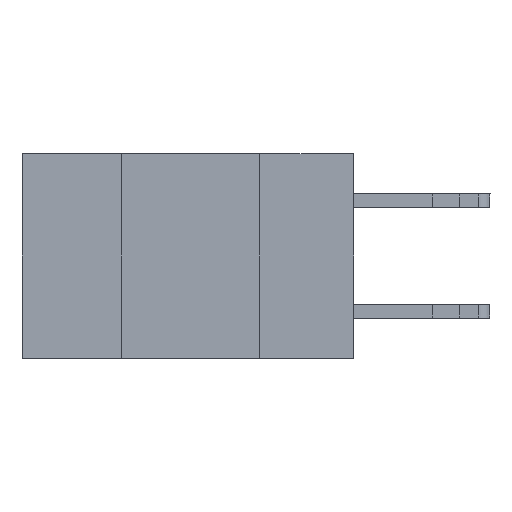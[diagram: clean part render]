
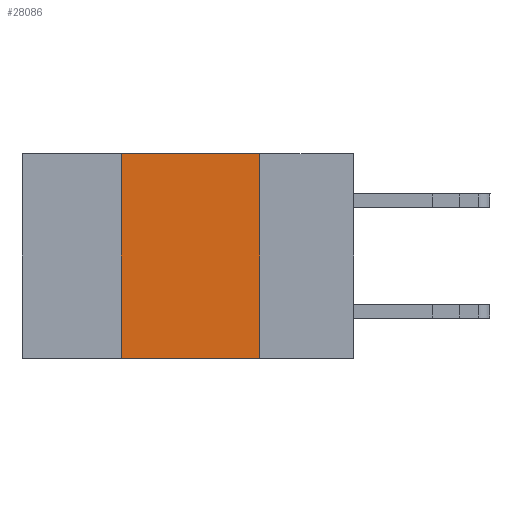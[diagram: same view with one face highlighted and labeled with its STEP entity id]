
A CAD part, left-side view. The second image highlights one B-rep face of the part: STEP entity #28086.
In plain terms, the highlighted planar face has unit normal (-1, 0, 0).
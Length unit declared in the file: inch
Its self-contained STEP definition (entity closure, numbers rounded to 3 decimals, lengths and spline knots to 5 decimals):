
#154 = DIRECTION ( 'NONE',  ( 0., -1., 0. ) ) ;
#2902 = CARTESIAN_POINT ( 'NONE',  ( 0., 0.17, 0. ) ) ;
#4293 = VERTEX_POINT ( 'NONE', #5622 ) ;
#4995 = DIRECTION ( 'NONE',  ( 0., 0., -1. ) ) ;
#5622 = CARTESIAN_POINT ( 'NONE',  ( 0., 0.42, 0. ) ) ;
#5686 = CARTESIAN_POINT ( 'NONE',  ( 0., 0.6, 0. ) ) ;
#6970 = VECTOR ( 'NONE', #25527, 39.37008 ) ;
#7393 = ORIENTED_EDGE ( 'NONE', *, *, #28038, .T. ) ;
#7588 = FACE_OUTER_BOUND ( 'NONE', #10348, .T. ) ;
#8051 = EDGE_CURVE ( 'NONE', #32552, #4293, #31285, .T. ) ;
#8640 = VERTEX_POINT ( 'NONE', #2902 ) ;
#9148 = AXIS2_PLACEMENT_3D ( 'NONE', #15513, #18278, #4995 ) ;
#9192 = ORIENTED_EDGE ( 'NONE', *, *, #17361, .F. ) ;
#10345 = LINE ( 'NONE', #5686, #25354 ) ;
#10348 = EDGE_LOOP ( 'NONE', ( #9192, #32559, #15653, #7393 ) ) ;
#15513 = CARTESIAN_POINT ( 'NONE',  ( 0., 0.6, 0. ) ) ;
#15522 = LINE ( 'NONE', #28818, #23710 ) ;
#15653 = ORIENTED_EDGE ( 'NONE', *, *, #8051, .F. ) ;
#15860 = DIRECTION ( 'NONE',  ( 0., 0., -1. ) ) ;
#17250 = CARTESIAN_POINT ( 'NONE',  ( 0., 0.6, -0.37 ) ) ;
#17361 = EDGE_CURVE ( 'NONE', #8640, #20488, #15522, .T. ) ;
#17445 = EDGE_CURVE ( 'NONE', #4293, #8640, #10345, .T. ) ;
#18278 = DIRECTION ( 'NONE',  ( 1., 0., 0. ) ) ;
#19264 = CARTESIAN_POINT ( 'NONE',  ( 0., 0.42, -0.37 ) ) ;
#20488 = VERTEX_POINT ( 'NONE', #31827 ) ;
#20576 = CARTESIAN_POINT ( 'NONE',  ( 0., 0.42, 0. ) ) ;
#22935 = PLANE ( 'NONE',  #9148 ) ;
#23710 = VECTOR ( 'NONE', #15860, 39.37008 ) ;
#25354 = VECTOR ( 'NONE', #154, 39.37008 ) ;
#25527 = DIRECTION ( 'NONE',  ( 0., -1., 0. ) ) ;
#25847 = VECTOR ( 'NONE', #26091, 39.37008 ) ;
#26091 = DIRECTION ( 'NONE',  ( 0., 0., 1. ) ) ;
#28038 = EDGE_CURVE ( 'NONE', #32552, #20488, #30721, .T. ) ;
#28086 = ADVANCED_FACE ( 'NONE', ( #7588 ), #22935, .F. ) ;
#28818 = CARTESIAN_POINT ( 'NONE',  ( 0., 0.17, 0. ) ) ;
#30721 = LINE ( 'NONE', #17250, #6970 ) ;
#31285 = LINE ( 'NONE', #20576, #25847 ) ;
#31827 = CARTESIAN_POINT ( 'NONE',  ( 0., 0.17, -0.37 ) ) ;
#32552 = VERTEX_POINT ( 'NONE', #19264 ) ;
#32559 = ORIENTED_EDGE ( 'NONE', *, *, #17445, .F. ) ;
